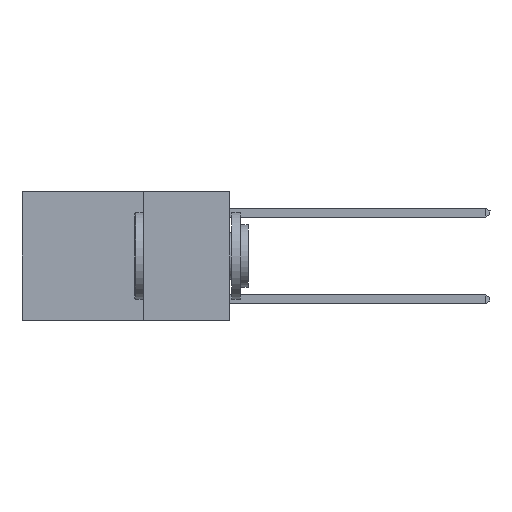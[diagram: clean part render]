
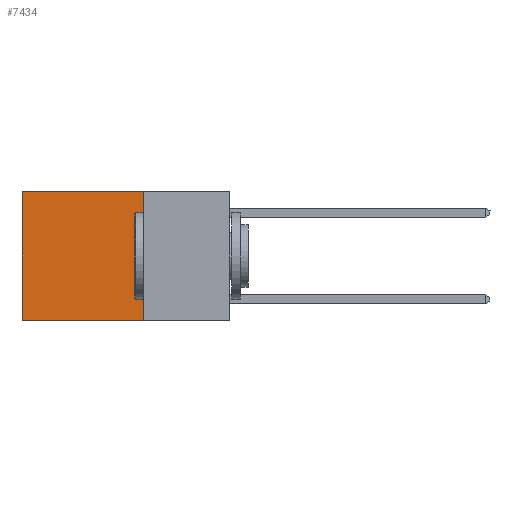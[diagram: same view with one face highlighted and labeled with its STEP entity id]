
A CAD part, left-side view. The second image highlights one B-rep face of the part: STEP entity #7434.
In plain terms, the highlighted planar face has unit normal (-1, 0, 0).
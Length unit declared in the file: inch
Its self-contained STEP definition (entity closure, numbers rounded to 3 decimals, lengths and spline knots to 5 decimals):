
#1685 = CARTESIAN_POINT ( 'NONE',  ( 0.2625, 0.25, 0. ) ) ;
#1756 = VECTOR ( 'NONE', #30673, 39.37008 ) ;
#3303 = VERTEX_POINT ( 'NONE', #28564 ) ;
#4562 = DIRECTION ( 'NONE',  ( 0., 1., 0. ) ) ;
#4872 = VERTEX_POINT ( 'NONE', #24402 ) ;
#5213 = VECTOR ( 'NONE', #4562, 39.37008 ) ;
#5835 = VERTEX_POINT ( 'NONE', #18483 ) ;
#7434 = ADVANCED_FACE ( 'NONE', ( #12773 ), #7950, .F. ) ;
#7950 = PLANE ( 'NONE',  #15849 ) ;
#9213 = DIRECTION ( 'NONE',  ( 0., 0., -1. ) ) ;
#10596 = ORIENTED_EDGE ( 'NONE', *, *, #13337, .F. ) ;
#11112 = ORIENTED_EDGE ( 'NONE', *, *, #21286, .T. ) ;
#11316 = LINE ( 'NONE', #23827, #22157 ) ;
#11676 = LINE ( 'NONE', #16786, #23823 ) ;
#12773 = FACE_OUTER_BOUND ( 'NONE', #17555, .T. ) ;
#13337 = EDGE_CURVE ( 'NONE', #17688, #5835, #11316, .T. ) ;
#13873 = CARTESIAN_POINT ( 'NONE',  ( 0.2625, 0.6, 0. ) ) ;
#15849 = AXIS2_PLACEMENT_3D ( 'NONE', #17735, #20292, #27648 ) ;
#15904 = ORIENTED_EDGE ( 'NONE', *, *, #20348, .T. ) ;
#16593 = LINE ( 'NONE', #13873, #1756 ) ;
#16786 = CARTESIAN_POINT ( 'NONE',  ( 0.2625, 0.25, 0. ) ) ;
#17555 = EDGE_LOOP ( 'NONE', ( #15904, #20957, #10596, #11112 ) ) ;
#17688 = VERTEX_POINT ( 'NONE', #1685 ) ;
#17735 = CARTESIAN_POINT ( 'NONE',  ( 0.2625, 0.25, 0. ) ) ;
#18483 = CARTESIAN_POINT ( 'NONE',  ( 0.2625, 0.25, -0.37 ) ) ;
#19470 = CARTESIAN_POINT ( 'NONE',  ( 0.2625, 0.25, -0.37 ) ) ;
#20292 = DIRECTION ( 'NONE',  ( 1., 0., 0. ) ) ;
#20348 = EDGE_CURVE ( 'NONE', #4872, #3303, #16593, .T. ) ;
#20957 = ORIENTED_EDGE ( 'NONE', *, *, #29885, .F. ) ;
#21286 = EDGE_CURVE ( 'NONE', #17688, #4872, #11676, .T. ) ;
#22157 = VECTOR ( 'NONE', #9213, 39.37008 ) ;
#23823 = VECTOR ( 'NONE', #28477, 39.37008 ) ;
#23827 = CARTESIAN_POINT ( 'NONE',  ( 0.2625, 0.25, 0. ) ) ;
#24402 = CARTESIAN_POINT ( 'NONE',  ( 0.2625, 0.6, 0. ) ) ;
#26508 = LINE ( 'NONE', #19470, #5213 ) ;
#27648 = DIRECTION ( 'NONE',  ( 0., 0., -1. ) ) ;
#28477 = DIRECTION ( 'NONE',  ( 0., 1., 0. ) ) ;
#28564 = CARTESIAN_POINT ( 'NONE',  ( 0.2625, 0.6, -0.37 ) ) ;
#29885 = EDGE_CURVE ( 'NONE', #5835, #3303, #26508, .T. ) ;
#30673 = DIRECTION ( 'NONE',  ( 0., 0., -1. ) ) ;
